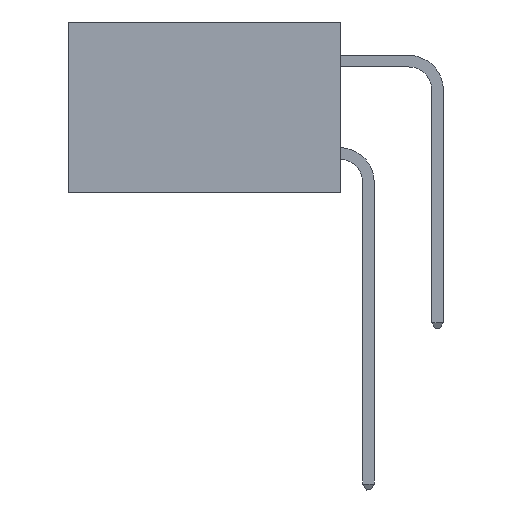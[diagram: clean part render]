
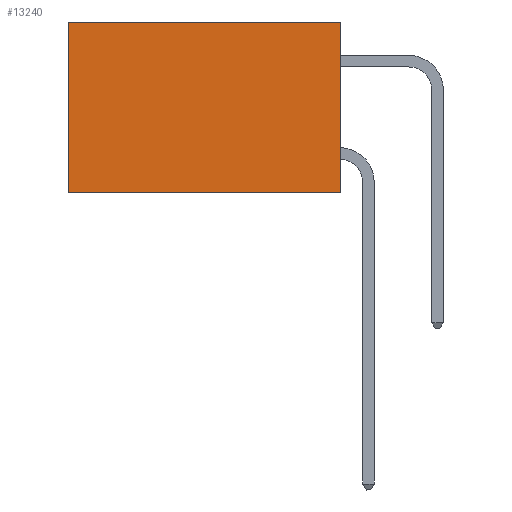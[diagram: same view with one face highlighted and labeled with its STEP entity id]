
A CAD part, left-side view. The second image highlights one B-rep face of the part: STEP entity #13240.
In plain terms, the highlighted planar face has unit normal (-1, 0, 0).
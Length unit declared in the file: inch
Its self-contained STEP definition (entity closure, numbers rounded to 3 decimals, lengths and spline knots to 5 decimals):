
#671 = PLANE ( 'NONE',  #34270 ) ;
#1629 = CARTESIAN_POINT ( 'NONE',  ( 0.277, 0., -0.37 ) ) ;
#1708 = DIRECTION ( 'NONE',  ( 0., 1., 0. ) ) ;
#2573 = VERTEX_POINT ( 'NONE', #25939 ) ;
#3459 = VECTOR ( 'NONE', #1708, 39.37008 ) ;
#3656 = EDGE_CURVE ( 'NONE', #2573, #3697, #3972, .T. ) ;
#3668 = EDGE_CURVE ( 'NONE', #2573, #29652, #17497, .T. ) ;
#3697 = VERTEX_POINT ( 'NONE', #9459 ) ;
#3972 = LINE ( 'NONE', #10387, #18359 ) ;
#4772 = EDGE_CURVE ( 'NONE', #3697, #6673, #10616, .T. ) ;
#5133 = CARTESIAN_POINT ( 'NONE',  ( 0.277, 0.59, -0.37 ) ) ;
#6093 = CARTESIAN_POINT ( 'NONE',  ( 0.277, 0., -0.37 ) ) ;
#6643 = ORIENTED_EDGE ( 'NONE', *, *, #3656, .F. ) ;
#6673 = VERTEX_POINT ( 'NONE', #5133 ) ;
#8065 = EDGE_CURVE ( 'NONE', #29652, #6673, #14211, .T. ) ;
#8780 = DIRECTION ( 'NONE',  ( 0., 0., -1. ) ) ;
#9459 = CARTESIAN_POINT ( 'NONE',  ( 0.277, 0., -0.37 ) ) ;
#9605 = CARTESIAN_POINT ( 'NONE',  ( 0.277, 0., 0. ) ) ;
#9734 = DIRECTION ( 'NONE',  ( 0., 0., -1. ) ) ;
#9934 = DIRECTION ( 'NONE',  ( 0., 1., 0. ) ) ;
#10387 = CARTESIAN_POINT ( 'NONE',  ( 0.277, 0., -0.37 ) ) ;
#10616 = LINE ( 'NONE', #1629, #3459 ) ;
#12123 = CARTESIAN_POINT ( 'NONE',  ( 0.277, 0.59, 0. ) ) ;
#13240 = ADVANCED_FACE ( 'NONE', ( #21038 ), #671, .F. ) ;
#13940 = ORIENTED_EDGE ( 'NONE', *, *, #3668, .T. ) ;
#14211 = LINE ( 'NONE', #19720, #33721 ) ;
#16996 = ORIENTED_EDGE ( 'NONE', *, *, #4772, .F. ) ;
#17497 = LINE ( 'NONE', #9605, #30742 ) ;
#18021 = ORIENTED_EDGE ( 'NONE', *, *, #8065, .T. ) ;
#18359 = VECTOR ( 'NONE', #9734, 39.37008 ) ;
#19720 = CARTESIAN_POINT ( 'NONE',  ( 0.277, 0.59, -0.37 ) ) ;
#21038 = FACE_OUTER_BOUND ( 'NONE', #33151, .T. ) ;
#21520 = DIRECTION ( 'NONE',  ( 0., 0., -1. ) ) ;
#24882 = DIRECTION ( 'NONE',  ( 1., 0., 0. ) ) ;
#25939 = CARTESIAN_POINT ( 'NONE',  ( 0.277, 0., 0. ) ) ;
#29652 = VERTEX_POINT ( 'NONE', #12123 ) ;
#30742 = VECTOR ( 'NONE', #9934, 39.37008 ) ;
#33151 = EDGE_LOOP ( 'NONE', ( #18021, #16996, #6643, #13940 ) ) ;
#33721 = VECTOR ( 'NONE', #21520, 39.37008 ) ;
#34270 = AXIS2_PLACEMENT_3D ( 'NONE', #6093, #24882, #8780 ) ;
